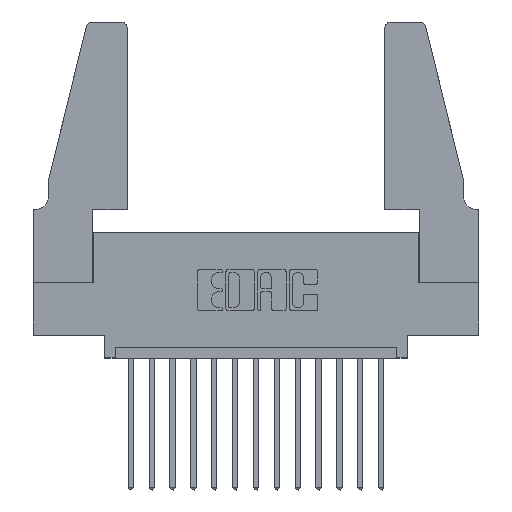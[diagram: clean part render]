
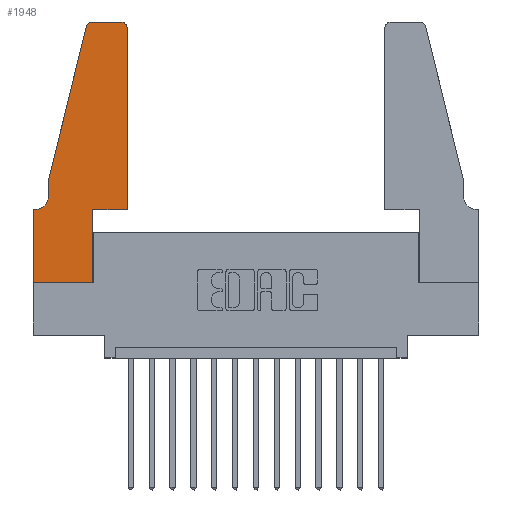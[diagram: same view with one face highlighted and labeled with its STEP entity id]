
A CAD part, top view. The second image highlights one B-rep face of the part: STEP entity #1948.
In plain terms, the highlighted planar face has unit normal (0, 0, 1).
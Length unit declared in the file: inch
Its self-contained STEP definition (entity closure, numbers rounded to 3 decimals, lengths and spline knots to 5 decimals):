
#8 = CARTESIAN_POINT ( 'NONE',  ( 0.284, 1.25, 0.37 ) ) ;
#88 = VERTEX_POINT ( 'NONE', #8471 ) ;
#264 = LINE ( 'NONE', #1086, #6483 ) ;
#333 = LINE ( 'NONE', #13230, #10054 ) ;
#661 = EDGE_CURVE ( 'NONE', #4783, #12003, #264, .T. ) ;
#765 = ORIENTED_EDGE ( 'NONE', *, *, #661, .T. ) ;
#862 = AXIS2_PLACEMENT_3D ( 'NONE', #15086, #2808, #1449 ) ;
#1086 = CARTESIAN_POINT ( 'NONE',  ( 0.0755, 0.5, 0.37 ) ) ;
#1110 = ORIENTED_EDGE ( 'NONE', *, *, #1894, .T. ) ;
#1213 = VECTOR ( 'NONE', #4677, 39.37008 ) ;
#1290 = CARTESIAN_POINT ( 'NONE',  ( 0.0755, 0.35, 0.37 ) ) ;
#1449 = DIRECTION ( 'NONE',  ( -1., 0., 0. ) ) ;
#1565 = ORIENTED_EDGE ( 'NONE', *, *, #5401, .T. ) ;
#1774 = DIRECTION ( 'NONE',  ( 0., 1., 0. ) ) ;
#1792 = VECTOR ( 'NONE', #3848, 39.37008 ) ;
#1894 = EDGE_CURVE ( 'NONE', #4861, #10607, #14698, .T. ) ;
#1948 = ADVANCED_FACE ( 'NONE', ( #12381 ), #15558, .T. ) ;
#2522 = ORIENTED_EDGE ( 'NONE', *, *, #11235, .T. ) ;
#2738 = VERTEX_POINT ( 'NONE', #3505 ) ;
#2808 = DIRECTION ( 'NONE',  ( 0., 0., -1. ) ) ;
#2825 = EDGE_CURVE ( 'NONE', #8337, #3711, #7183, .T. ) ;
#2863 = VECTOR ( 'NONE', #15411, 39.37008 ) ;
#3073 = DIRECTION ( 'NONE',  ( 1., 0., 0. ) ) ;
#3199 = VERTEX_POINT ( 'NONE', #15083 ) ;
#3221 = CARTESIAN_POINT ( 'NONE',  ( 0.0755, 0.42, 0.37 ) ) ;
#3478 = DIRECTION ( 'NONE',  ( 0., 1., 0. ) ) ;
#3505 = CARTESIAN_POINT ( 'NONE',  ( 0.0055, 0.35, 0.37 ) ) ;
#3539 = AXIS2_PLACEMENT_3D ( 'NONE', #12857, #5531, #11720 ) ;
#3711 = VERTEX_POINT ( 'NONE', #12523 ) ;
#3848 = DIRECTION ( 'NONE',  ( -1., 0., 0. ) ) ;
#3864 = CIRCLE ( 'NONE', #10410, 0.03 ) ;
#3866 = DIRECTION ( 'NONE',  ( 1., 0., 0. ) ) ;
#4505 = EDGE_CURVE ( 'NONE', #88, #4861, #333, .T. ) ;
#4544 = LINE ( 'NONE', #14149, #4937 ) ;
#4677 = DIRECTION ( 'NONE',  ( -0.239, -0.971, 0. ) ) ;
#4738 = EDGE_CURVE ( 'NONE', #11316, #88, #3864, .T. ) ;
#4783 = VERTEX_POINT ( 'NONE', #10832 ) ;
#4861 = VERTEX_POINT ( 'NONE', #8 ) ;
#4937 = VECTOR ( 'NONE', #1774, 39.37008 ) ;
#5043 = CARTESIAN_POINT ( 'NONE',  ( 0.2865, 0.35, 0.37 ) ) ;
#5195 = ORIENTED_EDGE ( 'NONE', *, *, #4505, .T. ) ;
#5401 = EDGE_CURVE ( 'NONE', #3711, #11503, #9429, .T. ) ;
#5479 = CARTESIAN_POINT ( 'NONE',  ( 0.284, 1.22, 0.37 ) ) ;
#5531 = DIRECTION ( 'NONE',  ( 0., 0., 1. ) ) ;
#5560 = CARTESIAN_POINT ( 'NONE',  ( 0., 0., 0.37 ) ) ;
#5934 = ORIENTED_EDGE ( 'NONE', *, *, #14804, .T. ) ;
#6087 = ORIENTED_EDGE ( 'NONE', *, *, #10136, .T. ) ;
#6291 = CARTESIAN_POINT ( 'NONE',  ( 0.4505, 0.35, 0.37 ) ) ;
#6483 = VECTOR ( 'NONE', #10955, 39.37008 ) ;
#6671 = EDGE_CURVE ( 'NONE', #3199, #11316, #4544, .T. ) ;
#7183 = LINE ( 'NONE', #13360, #11742 ) ;
#8239 = DIRECTION ( 'NONE',  ( 0., -1., 0. ) ) ;
#8337 = VERTEX_POINT ( 'NONE', #15084 ) ;
#8441 = DIRECTION ( 'NONE',  ( -1., 0., 0. ) ) ;
#8471 = CARTESIAN_POINT ( 'NONE',  ( 0.4205, 1.25, 0.37 ) ) ;
#9165 = ORIENTED_EDGE ( 'NONE', *, *, #6671, .T. ) ;
#9337 = LINE ( 'NONE', #14569, #1213 ) ;
#9429 = LINE ( 'NONE', #5560, #2863 ) ;
#9513 = EDGE_CURVE ( 'NONE', #11503, #15479, #12009, .T. ) ;
#9921 = EDGE_CURVE ( 'NONE', #2738, #8337, #14718, .T. ) ;
#10054 = VECTOR ( 'NONE', #8441, 39.37008 ) ;
#10136 = EDGE_CURVE ( 'NONE', #10607, #4783, #9337, .T. ) ;
#10314 = ORIENTED_EDGE ( 'NONE', *, *, #9513, .T. ) ;
#10410 = AXIS2_PLACEMENT_3D ( 'NONE', #12079, #10979, #11040 ) ;
#10419 = ORIENTED_EDGE ( 'NONE', *, *, #2825, .T. ) ;
#10487 = DIRECTION ( 'NONE',  ( 0., 0., 1. ) ) ;
#10607 = VERTEX_POINT ( 'NONE', #16012 ) ;
#10832 = CARTESIAN_POINT ( 'NONE',  ( 0.0755, 0.5, 0.37 ) ) ;
#10955 = DIRECTION ( 'NONE',  ( 0., -1., 0. ) ) ;
#10979 = DIRECTION ( 'NONE',  ( 0., 0., 1. ) ) ;
#11040 = DIRECTION ( 'NONE',  ( 1., 0., 0. ) ) ;
#11235 = EDGE_CURVE ( 'NONE', #15479, #3199, #12935, .T. ) ;
#11316 = VERTEX_POINT ( 'NONE', #13725 ) ;
#11423 = VECTOR ( 'NONE', #3866, 39.37008 ) ;
#11503 = VERTEX_POINT ( 'NONE', #15178 ) ;
#11648 = CIRCLE ( 'NONE', #862, 0.07 ) ;
#11720 = DIRECTION ( 'NONE',  ( 1., 0., 0. ) ) ;
#11742 = VECTOR ( 'NONE', #8239, 39.37008 ) ;
#12003 = VERTEX_POINT ( 'NONE', #3221 ) ;
#12009 = LINE ( 'NONE', #5043, #15685 ) ;
#12065 = AXIS2_PLACEMENT_3D ( 'NONE', #5479, #10487, #3073 ) ;
#12079 = CARTESIAN_POINT ( 'NONE',  ( 0.4205, 1.22, 0.37 ) ) ;
#12133 = ORIENTED_EDGE ( 'NONE', *, *, #4738, .T. ) ;
#12381 = FACE_OUTER_BOUND ( 'NONE', #14508, .T. ) ;
#12523 = CARTESIAN_POINT ( 'NONE',  ( 0., 0., 0.37 ) ) ;
#12857 = CARTESIAN_POINT ( 'NONE',  ( 0., 0.35, 0.37 ) ) ;
#12935 = LINE ( 'NONE', #6291, #11423 ) ;
#12997 = CARTESIAN_POINT ( 'NONE',  ( 0.2865, 0.35, 0.37 ) ) ;
#13230 = CARTESIAN_POINT ( 'NONE',  ( 0.2605, 1.25, 0.37 ) ) ;
#13360 = CARTESIAN_POINT ( 'NONE',  ( 0., 0., 0.37 ) ) ;
#13725 = CARTESIAN_POINT ( 'NONE',  ( 0.4505, 1.22, 0.37 ) ) ;
#14149 = CARTESIAN_POINT ( 'NONE',  ( 0.4505, 0.35, 0.37 ) ) ;
#14508 = EDGE_LOOP ( 'NONE', ( #5195, #1110, #6087, #765, #5934, #15536, #10419, #1565, #10314, #2522, #9165, #12133 ) ) ;
#14569 = CARTESIAN_POINT ( 'NONE',  ( 0.0755, 0.5, 0.37 ) ) ;
#14698 = CIRCLE ( 'NONE', #12065, 0.03 ) ;
#14718 = LINE ( 'NONE', #1290, #1792 ) ;
#14804 = EDGE_CURVE ( 'NONE', #12003, #2738, #11648, .T. ) ;
#15083 = CARTESIAN_POINT ( 'NONE',  ( 0.4505, 0.35, 0.37 ) ) ;
#15084 = CARTESIAN_POINT ( 'NONE',  ( 0., 0.35, 0.37 ) ) ;
#15086 = CARTESIAN_POINT ( 'NONE',  ( 0.0055, 0.42, 0.37 ) ) ;
#15178 = CARTESIAN_POINT ( 'NONE',  ( 0.2865, 0., 0.37 ) ) ;
#15411 = DIRECTION ( 'NONE',  ( 1., 0., 0. ) ) ;
#15479 = VERTEX_POINT ( 'NONE', #12997 ) ;
#15536 = ORIENTED_EDGE ( 'NONE', *, *, #9921, .T. ) ;
#15558 = PLANE ( 'NONE',  #3539 ) ;
#15685 = VECTOR ( 'NONE', #3478, 39.37008 ) ;
#16012 = CARTESIAN_POINT ( 'NONE',  ( 0.25487, 1.22718, 0.37 ) ) ;
